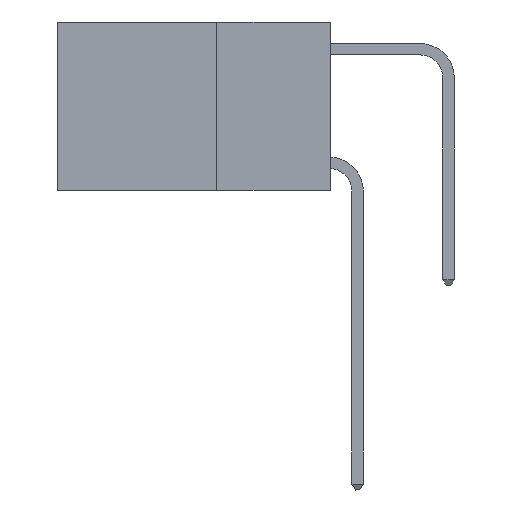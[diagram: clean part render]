
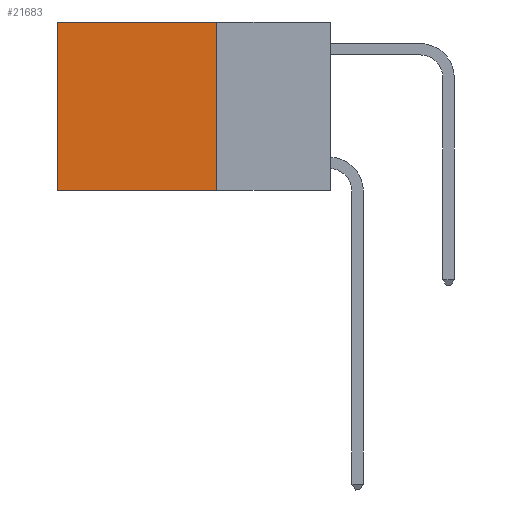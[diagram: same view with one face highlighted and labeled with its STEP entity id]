
A CAD part, left-side view. The second image highlights one B-rep face of the part: STEP entity #21683.
In plain terms, the highlighted planar face has unit normal (-1, 0, 0).
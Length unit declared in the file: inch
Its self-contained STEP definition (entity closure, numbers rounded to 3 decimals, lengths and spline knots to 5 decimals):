
#376 = EDGE_CURVE ( 'NONE', #18270, #7627, #21155, .T. ) ;
#402 = CARTESIAN_POINT ( 'NONE',  ( 0.2625, 0.6, 0. ) ) ;
#2633 = CARTESIAN_POINT ( 'NONE',  ( 0.2625, 0.25, -0.37 ) ) ;
#3463 = AXIS2_PLACEMENT_3D ( 'NONE', #17206, #20721, #8318 ) ;
#3676 = CARTESIAN_POINT ( 'NONE',  ( 0.2625, 0.25, 0. ) ) ;
#4244 = CARTESIAN_POINT ( 'NONE',  ( 0.2625, 0.25, 0. ) ) ;
#4925 = EDGE_CURVE ( 'NONE', #9423, #18270, #11399, .T. ) ;
#7386 = VERTEX_POINT ( 'NONE', #2633 ) ;
#7627 = VERTEX_POINT ( 'NONE', #23354 ) ;
#7773 = DIRECTION ( 'NONE',  ( 0., 0., -1. ) ) ;
#7846 = DIRECTION ( 'NONE',  ( 0., 1., 0. ) ) ;
#8252 = VECTOR ( 'NONE', #18838, 39.37008 ) ;
#8318 = DIRECTION ( 'NONE',  ( 0., 0., -1. ) ) ;
#9120 = VECTOR ( 'NONE', #9821, 39.37008 ) ;
#9423 = VERTEX_POINT ( 'NONE', #3676 ) ;
#9821 = DIRECTION ( 'NONE',  ( 0., 0., -1. ) ) ;
#9823 = EDGE_LOOP ( 'NONE', ( #18063, #20800, #11224, #14133 ) ) ;
#9942 = EDGE_CURVE ( 'NONE', #7386, #7627, #20742, .T. ) ;
#11224 = ORIENTED_EDGE ( 'NONE', *, *, #21156, .F. ) ;
#11399 = LINE ( 'NONE', #4244, #8252 ) ;
#11747 = CARTESIAN_POINT ( 'NONE',  ( 0.2625, 0.25, 0. ) ) ;
#12101 = LINE ( 'NONE', #11747, #9120 ) ;
#13637 = FACE_OUTER_BOUND ( 'NONE', #9823, .T. ) ;
#13834 = VECTOR ( 'NONE', #7846, 39.37008 ) ;
#14133 = ORIENTED_EDGE ( 'NONE', *, *, #4925, .T. ) ;
#14871 = VECTOR ( 'NONE', #7773, 39.37008 ) ;
#17206 = CARTESIAN_POINT ( 'NONE',  ( 0.2625, 0.25, 0. ) ) ;
#17567 = PLANE ( 'NONE',  #3463 ) ;
#18063 = ORIENTED_EDGE ( 'NONE', *, *, #376, .T. ) ;
#18270 = VERTEX_POINT ( 'NONE', #19003 ) ;
#18838 = DIRECTION ( 'NONE',  ( 0., 1., 0. ) ) ;
#19003 = CARTESIAN_POINT ( 'NONE',  ( 0.2625, 0.6, 0. ) ) ;
#20614 = CARTESIAN_POINT ( 'NONE',  ( 0.2625, 0.25, -0.37 ) ) ;
#20721 = DIRECTION ( 'NONE',  ( 1., 0., 0. ) ) ;
#20742 = LINE ( 'NONE', #20614, #13834 ) ;
#20800 = ORIENTED_EDGE ( 'NONE', *, *, #9942, .F. ) ;
#21155 = LINE ( 'NONE', #402, #14871 ) ;
#21156 = EDGE_CURVE ( 'NONE', #9423, #7386, #12101, .T. ) ;
#21683 = ADVANCED_FACE ( 'NONE', ( #13637 ), #17567, .F. ) ;
#23354 = CARTESIAN_POINT ( 'NONE',  ( 0.2625, 0.6, -0.37 ) ) ;
